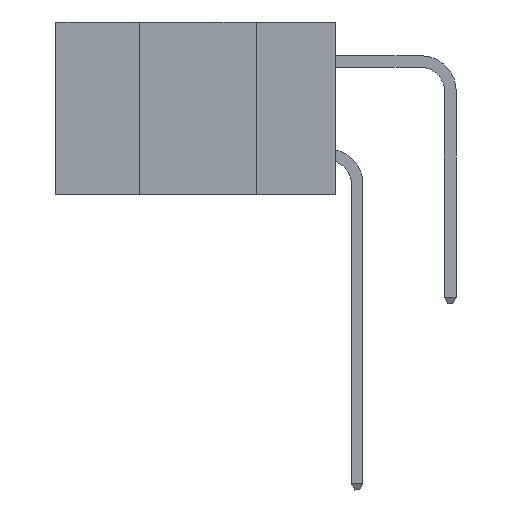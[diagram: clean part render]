
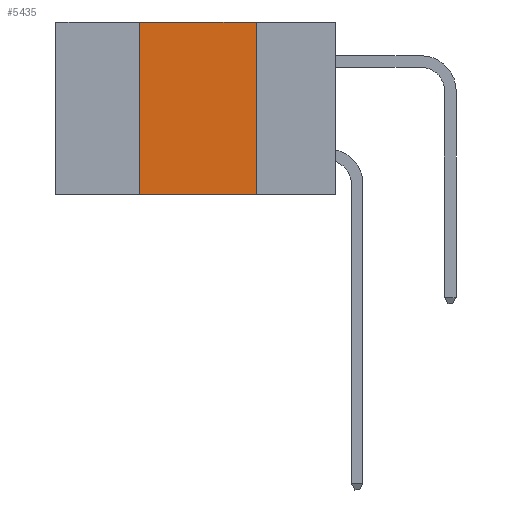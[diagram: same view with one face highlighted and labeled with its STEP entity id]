
A CAD part, left-side view. The second image highlights one B-rep face of the part: STEP entity #5435.
In plain terms, the highlighted planar face has unit normal (-1, 0, 0).
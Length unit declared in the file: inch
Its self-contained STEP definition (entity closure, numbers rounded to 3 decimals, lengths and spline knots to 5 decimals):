
#476 = CARTESIAN_POINT ( 'NONE',  ( 0., 0.42, 0. ) ) ;
#662 = LINE ( 'NONE', #2952, #9713 ) ;
#2349 = EDGE_CURVE ( 'NONE', #11816, #12663, #9513, .T. ) ;
#2486 = DIRECTION ( 'NONE',  ( 0., 0., 1. ) ) ;
#2952 = CARTESIAN_POINT ( 'NONE',  ( 0., 0.6, 0. ) ) ;
#3222 = DIRECTION ( 'NONE',  ( 0., -1., 0. ) ) ;
#4231 = VECTOR ( 'NONE', #21647, 39.37008 ) ;
#4791 = CARTESIAN_POINT ( 'NONE',  ( 0., 0.42, -0.37 ) ) ;
#5219 = FACE_OUTER_BOUND ( 'NONE', #9961, .T. ) ;
#5231 = DIRECTION ( 'NONE',  ( 0., 0., -1. ) ) ;
#5435 = ADVANCED_FACE ( 'NONE', ( #5219 ), #12672, .F. ) ;
#6262 = EDGE_CURVE ( 'NONE', #17035, #12663, #20700, .T. ) ;
#7120 = DIRECTION ( 'NONE',  ( 1., 0., 0. ) ) ;
#7651 = LINE ( 'NONE', #476, #19781 ) ;
#9513 = LINE ( 'NONE', #23159, #11406 ) ;
#9713 = VECTOR ( 'NONE', #3222, 39.37008 ) ;
#9938 = EDGE_CURVE ( 'NONE', #19893, #11816, #662, .T. ) ;
#9961 = EDGE_LOOP ( 'NONE', ( #20669, #14200, #11531, #16586 ) ) ;
#11406 = VECTOR ( 'NONE', #21277, 39.37008 ) ;
#11531 = ORIENTED_EDGE ( 'NONE', *, *, #19967, .F. ) ;
#11816 = VERTEX_POINT ( 'NONE', #25060 ) ;
#12093 = CARTESIAN_POINT ( 'NONE',  ( 0., 0.6, 0. ) ) ;
#12663 = VERTEX_POINT ( 'NONE', #23183 ) ;
#12672 = PLANE ( 'NONE',  #16069 ) ;
#13642 = CARTESIAN_POINT ( 'NONE',  ( 0., 0.6, -0.37 ) ) ;
#14200 = ORIENTED_EDGE ( 'NONE', *, *, #9938, .F. ) ;
#15599 = CARTESIAN_POINT ( 'NONE',  ( 0., 0.42, 0. ) ) ;
#16069 = AXIS2_PLACEMENT_3D ( 'NONE', #12093, #7120, #5231 ) ;
#16586 = ORIENTED_EDGE ( 'NONE', *, *, #6262, .T. ) ;
#17035 = VERTEX_POINT ( 'NONE', #4791 ) ;
#19781 = VECTOR ( 'NONE', #2486, 39.37008 ) ;
#19893 = VERTEX_POINT ( 'NONE', #15599 ) ;
#19967 = EDGE_CURVE ( 'NONE', #17035, #19893, #7651, .T. ) ;
#20669 = ORIENTED_EDGE ( 'NONE', *, *, #2349, .F. ) ;
#20700 = LINE ( 'NONE', #13642, #4231 ) ;
#21277 = DIRECTION ( 'NONE',  ( 0., 0., -1. ) ) ;
#21647 = DIRECTION ( 'NONE',  ( 0., -1., 0. ) ) ;
#23159 = CARTESIAN_POINT ( 'NONE',  ( 0., 0.17, 0. ) ) ;
#23183 = CARTESIAN_POINT ( 'NONE',  ( 0., 0.17, -0.37 ) ) ;
#25060 = CARTESIAN_POINT ( 'NONE',  ( 0., 0.17, 0. ) ) ;
